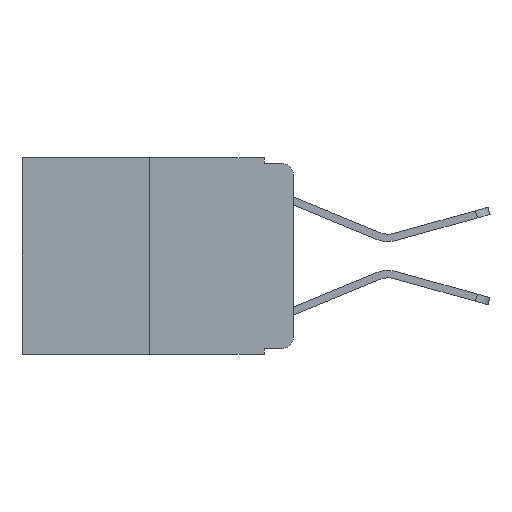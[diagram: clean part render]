
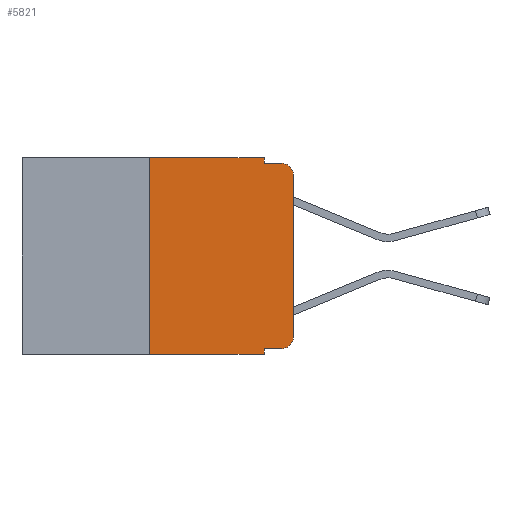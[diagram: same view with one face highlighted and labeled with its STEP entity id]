
A CAD part, left-side view. The second image highlights one B-rep face of the part: STEP entity #5821.
In plain terms, the highlighted planar face has unit normal (-1, 0, 0).
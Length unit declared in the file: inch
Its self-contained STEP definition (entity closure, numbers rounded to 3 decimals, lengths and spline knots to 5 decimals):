
#402 = LINE ( 'NONE', #3223, #5785 ) ;
#472 = VECTOR ( 'NONE', #11256, 39.37008 ) ;
#767 = AXIS2_PLACEMENT_3D ( 'NONE', #6894, #10556, #9895 ) ;
#781 = CARTESIAN_POINT ( 'NONE',  ( 0., 0.02, -0.01 ) ) ;
#868 = ORIENTED_EDGE ( 'NONE', *, *, #6228, .T. ) ;
#960 = EDGE_CURVE ( 'NONE', #10735, #10205, #3309, .T. ) ;
#1232 = VERTEX_POINT ( 'NONE', #11149 ) ;
#1290 = DIRECTION ( 'NONE',  ( -1., 0., 0. ) ) ;
#1334 = VECTOR ( 'NONE', #3078, 39.37008 ) ;
#1372 = DIRECTION ( 'NONE',  ( 0., 0., -1. ) ) ;
#1562 = ORIENTED_EDGE ( 'NONE', *, *, #5754, .F. ) ;
#1643 = DIRECTION ( 'NONE',  ( 0., 0., -1. ) ) ;
#1712 = VECTOR ( 'NONE', #3244, 39.37008 ) ;
#1899 = CARTESIAN_POINT ( 'NONE',  ( 0., 0., -0.03 ) ) ;
#2178 = CARTESIAN_POINT ( 'NONE',  ( 0., 0., 0. ) ) ;
#2555 = CARTESIAN_POINT ( 'NONE',  ( 0., 0.02, -0.03 ) ) ;
#2580 = LINE ( 'NONE', #6171, #9558 ) ;
#2662 = VECTOR ( 'NONE', #3028, 39.37008 ) ;
#2859 = CARTESIAN_POINT ( 'NONE',  ( 0., 0.25, 0. ) ) ;
#3028 = DIRECTION ( 'NONE',  ( 0., -1., 0. ) ) ;
#3035 = LINE ( 'NONE', #2859, #472 ) ;
#3078 = DIRECTION ( 'NONE',  ( 0., 0., 1. ) ) ;
#3148 = CARTESIAN_POINT ( 'NONE',  ( 0., 0.02, -0.333 ) ) ;
#3223 = CARTESIAN_POINT ( 'NONE',  ( 0., 0.473, 0. ) ) ;
#3232 = EDGE_CURVE ( 'NONE', #10830, #5864, #8371, .T. ) ;
#3244 = DIRECTION ( 'NONE',  ( 0., -1., 0. ) ) ;
#3309 = LINE ( 'NONE', #5154, #1712 ) ;
#3488 = EDGE_CURVE ( 'NONE', #10205, #10293, #10706, .T. ) ;
#3514 = EDGE_CURVE ( 'NONE', #11532, #5864, #6624, .T. ) ;
#3626 = DIRECTION ( 'NONE',  ( -1., 0., 0. ) ) ;
#3792 = EDGE_CURVE ( 'NONE', #10293, #10830, #3971, .T. ) ;
#3971 = LINE ( 'NONE', #2178, #1334 ) ;
#4186 = DIRECTION ( 'NONE',  ( 0., -1., 0. ) ) ;
#4319 = PLANE ( 'NONE',  #767 ) ;
#4389 = AXIS2_PLACEMENT_3D ( 'NONE', #2555, #3626, #1643 ) ;
#4451 = EDGE_CURVE ( 'NONE', #8267, #11532, #5924, .T. ) ;
#4981 = VECTOR ( 'NONE', #4186, 39.37008 ) ;
#5005 = DIRECTION ( 'NONE',  ( 0., 0., -1. ) ) ;
#5154 = CARTESIAN_POINT ( 'NONE',  ( 0., 0.051, -0.333 ) ) ;
#5213 = CARTESIAN_POINT ( 'NONE',  ( 0., 0.051, -0.333 ) ) ;
#5404 = CARTESIAN_POINT ( 'NONE',  ( 0., 0.051, -0.343 ) ) ;
#5654 = CARTESIAN_POINT ( 'NONE',  ( 0., 0.051, 0. ) ) ;
#5754 = EDGE_CURVE ( 'NONE', #10735, #9113, #2580, .T. ) ;
#5785 = VECTOR ( 'NONE', #8664, 39.37008 ) ;
#5821 = ADVANCED_FACE ( 'NONE', ( #8003 ), #4319, .F. ) ;
#5864 = VERTEX_POINT ( 'NONE', #781 ) ;
#5924 = LINE ( 'NONE', #7885, #6316 ) ;
#6093 = CARTESIAN_POINT ( 'NONE',  ( 0., 0.473, -0.343 ) ) ;
#6171 = CARTESIAN_POINT ( 'NONE',  ( 0., 0.051, 0. ) ) ;
#6228 = EDGE_CURVE ( 'NONE', #1232, #9113, #9827, .T. ) ;
#6316 = VECTOR ( 'NONE', #1372, 39.37008 ) ;
#6405 = ORIENTED_EDGE ( 'NONE', *, *, #3232, .T. ) ;
#6624 = LINE ( 'NONE', #11374, #2662 ) ;
#6841 = EDGE_LOOP ( 'NONE', ( #7481, #6405, #8834, #10748, #7696, #11489, #868, #1562, #10272, #8343 ) ) ;
#6894 = CARTESIAN_POINT ( 'NONE',  ( 0., 0.473, 0. ) ) ;
#6950 = DIRECTION ( 'NONE',  ( 0., 0., -1. ) ) ;
#6967 = CARTESIAN_POINT ( 'NONE',  ( 0., 0.25, 0. ) ) ;
#7098 = VERTEX_POINT ( 'NONE', #6967 ) ;
#7481 = ORIENTED_EDGE ( 'NONE', *, *, #3792, .T. ) ;
#7696 = ORIENTED_EDGE ( 'NONE', *, *, #8035, .F. ) ;
#7885 = CARTESIAN_POINT ( 'NONE',  ( 0., 0.051, 0. ) ) ;
#8003 = FACE_OUTER_BOUND ( 'NONE', #6841, .T. ) ;
#8035 = EDGE_CURVE ( 'NONE', #7098, #8267, #402, .T. ) ;
#8267 = VERTEX_POINT ( 'NONE', #5654 ) ;
#8343 = ORIENTED_EDGE ( 'NONE', *, *, #3488, .T. ) ;
#8371 = CIRCLE ( 'NONE', #4389, 0.02 ) ;
#8588 = CARTESIAN_POINT ( 'NONE',  ( 0., 0.051, -0.01 ) ) ;
#8664 = DIRECTION ( 'NONE',  ( 0., -1., 0. ) ) ;
#8748 = CARTESIAN_POINT ( 'NONE',  ( 0., 0., -0.313 ) ) ;
#8834 = ORIENTED_EDGE ( 'NONE', *, *, #3514, .F. ) ;
#8970 = AXIS2_PLACEMENT_3D ( 'NONE', #9491, #1290, #5005 ) ;
#9113 = VERTEX_POINT ( 'NONE', #5404 ) ;
#9491 = CARTESIAN_POINT ( 'NONE',  ( 0., 0.02, -0.313 ) ) ;
#9558 = VECTOR ( 'NONE', #6950, 39.37008 ) ;
#9827 = LINE ( 'NONE', #6093, #4981 ) ;
#9895 = DIRECTION ( 'NONE',  ( 0., 0., -1. ) ) ;
#10205 = VERTEX_POINT ( 'NONE', #3148 ) ;
#10272 = ORIENTED_EDGE ( 'NONE', *, *, #960, .T. ) ;
#10293 = VERTEX_POINT ( 'NONE', #8748 ) ;
#10556 = DIRECTION ( 'NONE',  ( 1., 0., 0. ) ) ;
#10706 = CIRCLE ( 'NONE', #8970, 0.02 ) ;
#10735 = VERTEX_POINT ( 'NONE', #5213 ) ;
#10748 = ORIENTED_EDGE ( 'NONE', *, *, #4451, .F. ) ;
#10830 = VERTEX_POINT ( 'NONE', #1899 ) ;
#11149 = CARTESIAN_POINT ( 'NONE',  ( 0., 0.25, -0.343 ) ) ;
#11256 = DIRECTION ( 'NONE',  ( 0., 0., 1. ) ) ;
#11374 = CARTESIAN_POINT ( 'NONE',  ( 0., 0.051, -0.01 ) ) ;
#11489 = ORIENTED_EDGE ( 'NONE', *, *, #11775, .F. ) ;
#11532 = VERTEX_POINT ( 'NONE', #8588 ) ;
#11775 = EDGE_CURVE ( 'NONE', #1232, #7098, #3035, .T. ) ;
